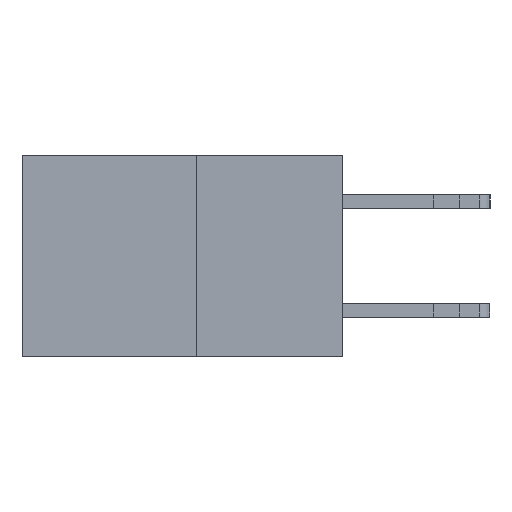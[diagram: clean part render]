
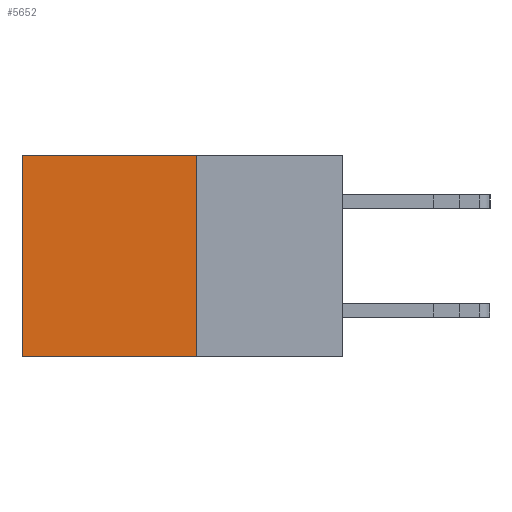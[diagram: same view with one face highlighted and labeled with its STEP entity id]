
A CAD part, left-side view. The second image highlights one B-rep face of the part: STEP entity #5652.
In plain terms, the highlighted planar face has unit normal (-1, 0, 0).
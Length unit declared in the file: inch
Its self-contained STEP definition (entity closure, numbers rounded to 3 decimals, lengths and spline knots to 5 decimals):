
#17 = CARTESIAN_POINT ( 'NONE',  ( 0.277, 0.59, -0.37 ) ) ;
#233 = VECTOR ( 'NONE', #8250, 39.37008 ) ;
#397 = EDGE_CURVE ( 'NONE', #14713, #8913, #12767, .T. ) ;
#655 = PLANE ( 'NONE',  #8894 ) ;
#1193 = EDGE_CURVE ( 'NONE', #13133, #8913, #6221, .T. ) ;
#1744 = VECTOR ( 'NONE', #10929, 39.37008 ) ;
#1865 = DIRECTION ( 'NONE',  ( 0., 0., -1. ) ) ;
#2124 = LINE ( 'NONE', #2719, #1744 ) ;
#2719 = CARTESIAN_POINT ( 'NONE',  ( 0.277, 0.27, -0.37 ) ) ;
#3703 = CARTESIAN_POINT ( 'NONE',  ( 0.277, 0.27, -0.37 ) ) ;
#3891 = DIRECTION ( 'NONE',  ( 0., 1., 0. ) ) ;
#4246 = EDGE_LOOP ( 'NONE', ( #11784, #12305, #14966, #5783 ) ) ;
#4247 = CARTESIAN_POINT ( 'NONE',  ( 0.277, 0.59, 0. ) ) ;
#5327 = VERTEX_POINT ( 'NONE', #8340 ) ;
#5521 = LINE ( 'NONE', #8553, #14019 ) ;
#5652 = ADVANCED_FACE ( 'NONE', ( #15125 ), #655, .F. ) ;
#5783 = ORIENTED_EDGE ( 'NONE', *, *, #6665, .T. ) ;
#6221 = LINE ( 'NONE', #8167, #233 ) ;
#6665 = EDGE_CURVE ( 'NONE', #5327, #14713, #5521, .T. ) ;
#7780 = CARTESIAN_POINT ( 'NONE',  ( 0.277, 0.27, -0.37 ) ) ;
#8167 = CARTESIAN_POINT ( 'NONE',  ( 0.277, 0.27, -0.37 ) ) ;
#8250 = DIRECTION ( 'NONE',  ( 0., 1., 0. ) ) ;
#8340 = CARTESIAN_POINT ( 'NONE',  ( 0.277, 0.27, 0. ) ) ;
#8450 = EDGE_CURVE ( 'NONE', #5327, #13133, #2124, .T. ) ;
#8553 = CARTESIAN_POINT ( 'NONE',  ( 0.277, 0.27, 0. ) ) ;
#8894 = AXIS2_PLACEMENT_3D ( 'NONE', #7780, #8931, #1865 ) ;
#8913 = VERTEX_POINT ( 'NONE', #14009 ) ;
#8931 = DIRECTION ( 'NONE',  ( 1., 0., 0. ) ) ;
#9711 = VECTOR ( 'NONE', #15104, 39.37008 ) ;
#10929 = DIRECTION ( 'NONE',  ( 0., 0., -1. ) ) ;
#11784 = ORIENTED_EDGE ( 'NONE', *, *, #397, .T. ) ;
#12305 = ORIENTED_EDGE ( 'NONE', *, *, #1193, .F. ) ;
#12767 = LINE ( 'NONE', #17, #9711 ) ;
#13133 = VERTEX_POINT ( 'NONE', #3703 ) ;
#14009 = CARTESIAN_POINT ( 'NONE',  ( 0.277, 0.59, -0.37 ) ) ;
#14019 = VECTOR ( 'NONE', #3891, 39.37008 ) ;
#14713 = VERTEX_POINT ( 'NONE', #4247 ) ;
#14966 = ORIENTED_EDGE ( 'NONE', *, *, #8450, .F. ) ;
#15104 = DIRECTION ( 'NONE',  ( 0., 0., -1. ) ) ;
#15125 = FACE_OUTER_BOUND ( 'NONE', #4246, .T. ) ;
